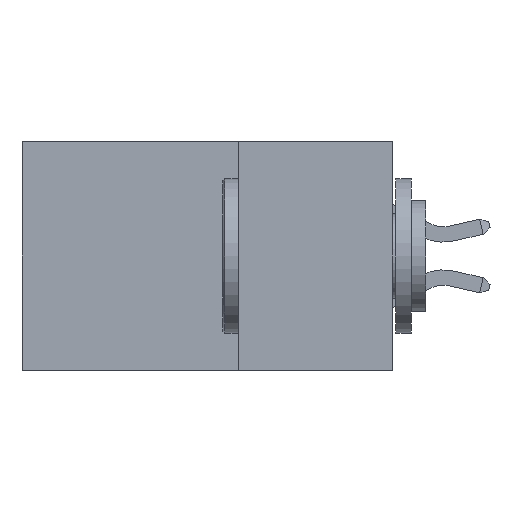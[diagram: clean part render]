
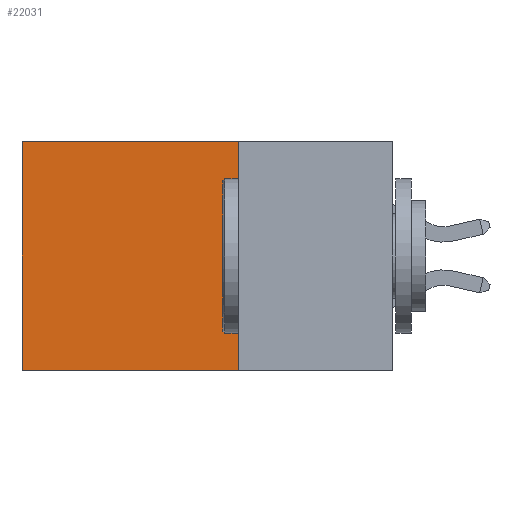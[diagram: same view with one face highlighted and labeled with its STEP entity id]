
A CAD part, left-side view. The second image highlights one B-rep face of the part: STEP entity #22031.
In plain terms, the highlighted planar face has unit normal (-1, 0, 0).
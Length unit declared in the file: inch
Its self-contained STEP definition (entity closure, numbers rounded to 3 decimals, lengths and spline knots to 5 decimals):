
#1499 = AXIS2_PLACEMENT_3D ( 'NONE', #25940, #11143, #2475 ) ;
#2013 = ORIENTED_EDGE ( 'NONE', *, *, #21036, .T. ) ;
#2475 = DIRECTION ( 'NONE',  ( 0., 0., -1. ) ) ;
#2558 = EDGE_CURVE ( 'NONE', #30743, #8985, #35884, .T. ) ;
#5188 = ORIENTED_EDGE ( 'NONE', *, *, #2558, .F. ) ;
#5765 = LINE ( 'NONE', #30055, #37191 ) ;
#5986 = EDGE_CURVE ( 'NONE', #22298, #30743, #23922, .T. ) ;
#6035 = CARTESIAN_POINT ( 'NONE',  ( 0.2875, 0.25, 0. ) ) ;
#7200 = DIRECTION ( 'NONE',  ( 0., 0., -1. ) ) ;
#8985 = VERTEX_POINT ( 'NONE', #27408 ) ;
#9555 = DIRECTION ( 'NONE',  ( 0., 1., 0. ) ) ;
#11143 = DIRECTION ( 'NONE',  ( 1., 0., 0. ) ) ;
#12198 = VECTOR ( 'NONE', #22080, 39.37008 ) ;
#13072 = CARTESIAN_POINT ( 'NONE',  ( 0.2875, 0.25, -0.37 ) ) ;
#15506 = DIRECTION ( 'NONE',  ( 0., 0., -1. ) ) ;
#17310 = EDGE_CURVE ( 'NONE', #32360, #8985, #5765, .T. ) ;
#20389 = VECTOR ( 'NONE', #9555, 39.37008 ) ;
#20922 = ORIENTED_EDGE ( 'NONE', *, *, #5986, .F. ) ;
#21036 = EDGE_CURVE ( 'NONE', #22298, #32360, #28143, .T. ) ;
#21584 = CARTESIAN_POINT ( 'NONE',  ( 0.2875, 0.25, -0.37 ) ) ;
#21600 = VECTOR ( 'NONE', #7200, 39.37008 ) ;
#21686 = FACE_OUTER_BOUND ( 'NONE', #26995, .T. ) ;
#22031 = ADVANCED_FACE ( 'NONE', ( #21686 ), #23024, .F. ) ;
#22080 = DIRECTION ( 'NONE',  ( 0., 1., 0. ) ) ;
#22298 = VERTEX_POINT ( 'NONE', #6035 ) ;
#22552 = ORIENTED_EDGE ( 'NONE', *, *, #17310, .T. ) ;
#23024 = PLANE ( 'NONE',  #1499 ) ;
#23922 = LINE ( 'NONE', #30380, #21600 ) ;
#24095 = CARTESIAN_POINT ( 'NONE',  ( 0.2875, 0.6, 0. ) ) ;
#25940 = CARTESIAN_POINT ( 'NONE',  ( 0.2875, 0.25, 0. ) ) ;
#26995 = EDGE_LOOP ( 'NONE', ( #22552, #5188, #20922, #2013 ) ) ;
#27408 = CARTESIAN_POINT ( 'NONE',  ( 0.2875, 0.6, -0.37 ) ) ;
#28143 = LINE ( 'NONE', #32858, #20389 ) ;
#30055 = CARTESIAN_POINT ( 'NONE',  ( 0.2875, 0.6, 0. ) ) ;
#30380 = CARTESIAN_POINT ( 'NONE',  ( 0.2875, 0.25, 0. ) ) ;
#30743 = VERTEX_POINT ( 'NONE', #13072 ) ;
#32360 = VERTEX_POINT ( 'NONE', #24095 ) ;
#32858 = CARTESIAN_POINT ( 'NONE',  ( 0.2875, 0.25, 0. ) ) ;
#35884 = LINE ( 'NONE', #21584, #12198 ) ;
#37191 = VECTOR ( 'NONE', #15506, 39.37008 ) ;
